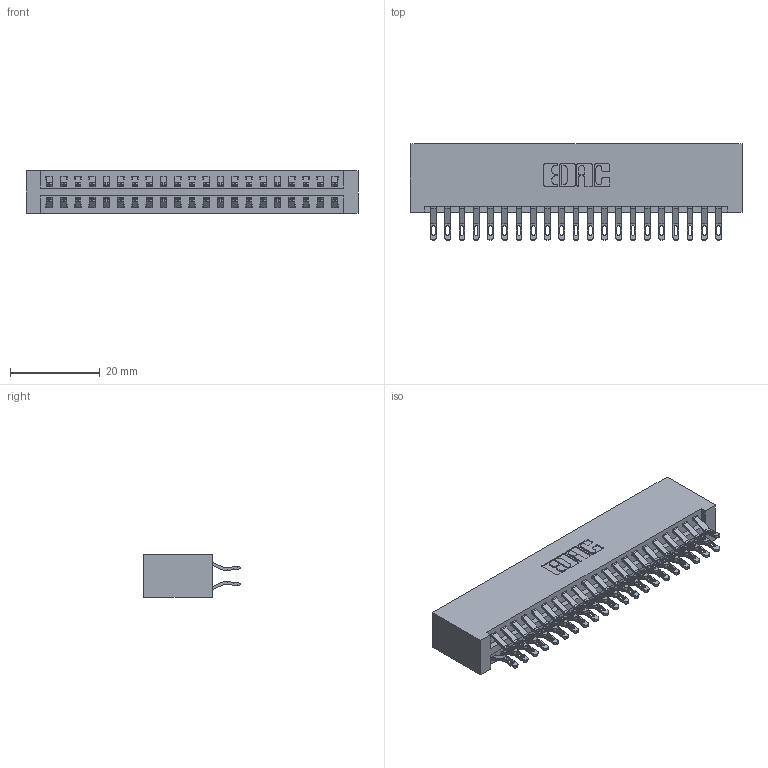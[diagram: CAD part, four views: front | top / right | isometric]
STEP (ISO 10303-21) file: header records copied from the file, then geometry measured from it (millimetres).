
FILE_DESCRIPTION (( 'STEP AP203' ), '1' );
FILE_NAME ('346-042-555-201.STEP', '2018-08-24T22:51:38', ( '' ), ( '' ), 'SwSTEP 2.0', 'SolidWorks 2016', '' );
FILE_SCHEMA (( 'CONFIG_CONTROL_DESIGN' ));
Length unit declared in the file: inch
Products named in the file (3): 346 Part_No Mounting Lugs; 345-292-001_555 Tail; 346-042-555-201
Assembly tree (43 placements, depth 2):
  346-042-555-201
    346 Part_No Mounting Lugs
    345-292-001_555 Tail  x42
Bounding box: 73.91 x 21.46 x 9.4 mm (x, y, z)
Volume: 7739.5 mm3; surface area: 10905.9 mm2
Topology: 43 solids, 43 shells, 2550 faces, 7991 edges, 5326 vertices
Faces by surface type: plane 1458, cylinder 1092
Entity records: 16581 total; most frequent: CARTESIAN_POINT 2794, ORIENTED_EDGE 2698, DIRECTION 2477, EDGE_CURVE 1349, LINE 1121, VECTOR 1121, VERTEX_POINT 898, AXIS2_PLACEMENT_3D 678
